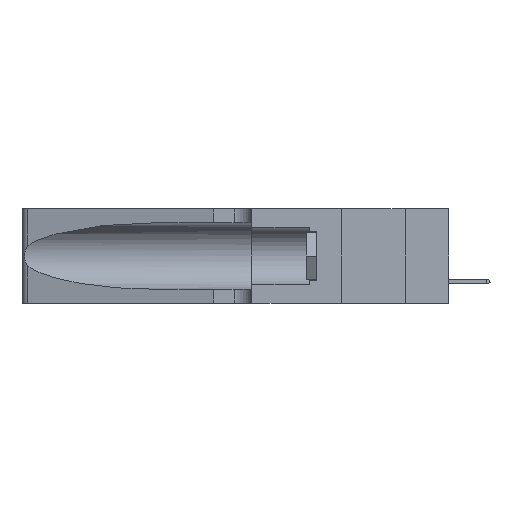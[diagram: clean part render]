
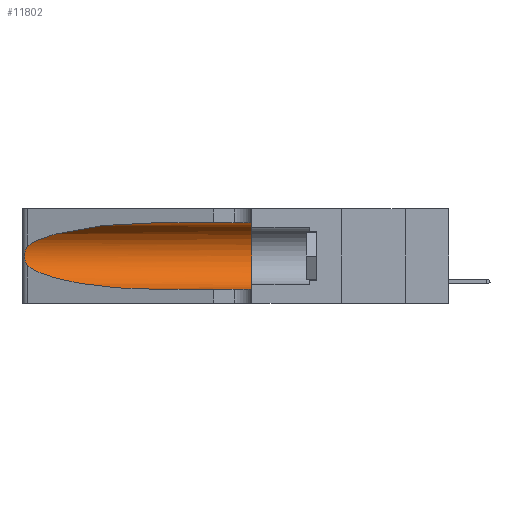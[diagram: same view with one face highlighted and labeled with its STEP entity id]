
A CAD part, left-side view. The second image highlights one B-rep face of the part: STEP entity #11802.
In plain terms, the highlighted cylindrical face has radius 3.308 mm (diameter 6.617 mm), a partial arc.
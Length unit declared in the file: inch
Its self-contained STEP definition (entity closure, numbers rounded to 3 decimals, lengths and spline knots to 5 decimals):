
#391 = CARTESIAN_POINT ( 'NONE',  ( 0.18966, 0.96281, 0.05475 ) ) ;
#910 = CARTESIAN_POINT ( 'NONE',  ( 0.25787, 1.23484, 0.2124 ) ) ;
#1155 =( BOUNDED_CURVE ( )  B_SPLINE_CURVE ( 3, ( #16851, #19258, #17045, #21481 ),
 .UNSPECIFIED., .F., .F. ) 
 B_SPLINE_CURVE_WITH_KNOTS ( ( 4, 4 ),
 ( 1.5708, 2.84003 ),
 .UNSPECIFIED. ) 
 CURVE ( )  GEOMETRIC_REPRESENTATION_ITEM ( )  RATIONAL_B_SPLINE_CURVE ( ( 1., 0.87, 0.87, 1. ) ) 
 REPRESENTATION_ITEM ( '' )  );
#1519 = CARTESIAN_POINT ( 'NONE',  ( 0.1305, 1.61858, 0.05475 ) ) ;
#2361 = AXIS2_PLACEMENT_3D ( 'NONE', #5373, #2855, #23824 ) ;
#2500 = EDGE_CURVE ( 'NONE', #5797, #26246, #19290, .T. ) ;
#2855 = DIRECTION ( 'NONE',  ( 0., -1., 0. ) ) ;
#3174 = DIRECTION ( 'NONE',  ( 0., 1., 0. ) ) ;
#3616 = CARTESIAN_POINT ( 'NONE',  ( 0.26017, 1.23833, 0.17102 ) ) ;
#3921 = CIRCLE ( 'NONE', #14284, 0.13025 ) ;
#5373 = CARTESIAN_POINT ( 'NONE',  ( 0.1305, 1.61858, 0.185 ) ) ;
#5780 = DIRECTION ( 'NONE',  ( 0., -1., 0. ) ) ;
#5797 = VERTEX_POINT ( 'NONE', #12887 ) ;
#6040 = LINE ( 'NONE', #1519, #25731 ) ;
#6137 = CARTESIAN_POINT ( 'NONE',  ( 0.1305, 0.72297, 0.05475 ) ) ;
#6243 = CARTESIAN_POINT ( 'NONE',  ( 0.1305, 0.35, 0.185 ) ) ;
#7071 = CARTESIAN_POINT ( 'NONE',  ( 0.25487, 1.22718, 0.22369 ) ) ;
#7083 = EDGE_LOOP ( 'NONE', ( #22136, #16729, #14501, #23531, #12642, #26061 ) ) ;
#8078 = DIRECTION ( 'NONE',  ( 0., -1., 0. ) ) ;
#8560 = CARTESIAN_POINT ( 'NONE',  ( 0.25487, 1.22718, 0.14631 ) ) ;
#9468 = CARTESIAN_POINT ( 'NONE',  ( 0.25555, 1.22994, 0.2215 ) ) ;
#9824 = VERTEX_POINT ( 'NONE', #27220 ) ;
#10405 = CARTESIAN_POINT ( 'NONE',  ( 0.25487, 1.22718, 0.14631 ) ) ;
#10604 = CARTESIAN_POINT ( 'NONE',  ( 0.25789, 1.23486, 0.15765 ) ) ;
#11284 = EDGE_CURVE ( 'NONE', #9824, #5797, #1155, .T. ) ;
#11376 = CARTESIAN_POINT ( 'NONE',  ( 0.1305, 0.35, 0.31525 ) ) ;
#11459 = VECTOR ( 'NONE', #5780, 39.37008 ) ;
#11513 = CARTESIAN_POINT ( 'NONE',  ( 0.25487, 1.22718, 0.14631 ) ) ;
#11802 = ADVANCED_FACE ( 'NONE', ( #12704 ), #14123, .F. ) ;
#11998 = CARTESIAN_POINT ( 'NONE',  ( 0.2373, 1.15595, 0.08982 ) ) ;
#12642 = ORIENTED_EDGE ( 'NONE', *, *, #20028, .F. ) ;
#12703 =( BOUNDED_CURVE ( )  B_SPLINE_CURVE ( 3, ( #11513, #11998, #391, #28132 ),
 .UNSPECIFIED., .F., .F. ) 
 B_SPLINE_CURVE_WITH_KNOTS ( ( 4, 4 ),
 ( 3.44316, 4.71239 ),
 .UNSPECIFIED. ) 
 CURVE ( )  GEOMETRIC_REPRESENTATION_ITEM ( )  RATIONAL_B_SPLINE_CURVE ( ( 1., 0.87, 0.87, 1. ) ) 
 REPRESENTATION_ITEM ( '' )  );
#12704 = FACE_OUTER_BOUND ( 'NONE', #7083, .T. ) ;
#12887 = CARTESIAN_POINT ( 'NONE',  ( 0.25487, 1.22718, 0.22369 ) ) ;
#13257 = EDGE_CURVE ( 'NONE', #26246, #16167, #12703, .T. ) ;
#13560 = CARTESIAN_POINT ( 'NONE',  ( 0.1305, 0.35, 0.05475 ) ) ;
#14123 = CYLINDRICAL_SURFACE ( 'NONE', #2361, 0.13025 ) ;
#14284 = AXIS2_PLACEMENT_3D ( 'NONE', #6243, #3174, #23210 ) ;
#14501 = ORIENTED_EDGE ( 'NONE', *, *, #13257, .T. ) ;
#15106 = CARTESIAN_POINT ( 'NONE',  ( 0.26075, 1.23896, 0.19203 ) ) ;
#16167 = VERTEX_POINT ( 'NONE', #6137 ) ;
#16476 = CARTESIAN_POINT ( 'NONE',  ( 0.25639, 1.23184, 0.21858 ) ) ;
#16729 = ORIENTED_EDGE ( 'NONE', *, *, #2500, .T. ) ;
#16851 = CARTESIAN_POINT ( 'NONE',  ( 0.1305, 0.72297, 0.31525 ) ) ;
#17045 = CARTESIAN_POINT ( 'NONE',  ( 0.2373, 1.15595, 0.28018 ) ) ;
#19258 = CARTESIAN_POINT ( 'NONE',  ( 0.18966, 0.96281, 0.31525 ) ) ;
#19290 = B_SPLINE_CURVE_WITH_KNOTS ( 'NONE', 3,
 ( #7071, #9468, #16476, #910, #23955, #26543, #15106, #19897, #3616, #19695, #10604, #26852, #22153, #10405 ),
 .UNSPECIFIED., .F., .F.,
 ( 4, 2, 2, 2, 2, 2, 4 ),
 ( 0., 0.00027, 0.00053, 0.00107, 0.0016, 0.00187, 0.00214 ),
 .UNSPECIFIED. ) ;
#19695 = CARTESIAN_POINT ( 'NONE',  ( 0.25856, 1.23593, 0.16098 ) ) ;
#19699 = LINE ( 'NONE', #28392, #11459 ) ;
#19897 = CARTESIAN_POINT ( 'NONE',  ( 0.26075, 1.23896, 0.178 ) ) ;
#20028 = EDGE_CURVE ( 'NONE', #28910, #27679, #3921, .T. ) ;
#20208 = EDGE_CURVE ( 'NONE', #16167, #27679, #6040, .T. ) ;
#21481 = CARTESIAN_POINT ( 'NONE',  ( 0.25487, 1.22718, 0.22369 ) ) ;
#22136 = ORIENTED_EDGE ( 'NONE', *, *, #11284, .T. ) ;
#22153 = CARTESIAN_POINT ( 'NONE',  ( 0.25555, 1.22993, 0.14849 ) ) ;
#23210 = DIRECTION ( 'NONE',  ( 0., 0., 1. ) ) ;
#23236 = EDGE_CURVE ( 'NONE', #9824, #28910, #19699, .T. ) ;
#23531 = ORIENTED_EDGE ( 'NONE', *, *, #20208, .T. ) ;
#23824 = DIRECTION ( 'NONE',  ( 0., 0., -1. ) ) ;
#23955 = CARTESIAN_POINT ( 'NONE',  ( 0.25854, 1.2359, 0.20912 ) ) ;
#25731 = VECTOR ( 'NONE', #8078, 39.37008 ) ;
#26061 = ORIENTED_EDGE ( 'NONE', *, *, #23236, .F. ) ;
#26246 = VERTEX_POINT ( 'NONE', #8560 ) ;
#26543 = CARTESIAN_POINT ( 'NONE',  ( 0.26018, 1.23835, 0.19895 ) ) ;
#26852 = CARTESIAN_POINT ( 'NONE',  ( 0.25639, 1.23186, 0.15144 ) ) ;
#27220 = CARTESIAN_POINT ( 'NONE',  ( 0.1305, 0.72297, 0.31525 ) ) ;
#27679 = VERTEX_POINT ( 'NONE', #13560 ) ;
#28132 = CARTESIAN_POINT ( 'NONE',  ( 0.1305, 0.72297, 0.05475 ) ) ;
#28392 = CARTESIAN_POINT ( 'NONE',  ( 0.1305, 1.61858, 0.31525 ) ) ;
#28910 = VERTEX_POINT ( 'NONE', #11376 ) ;
